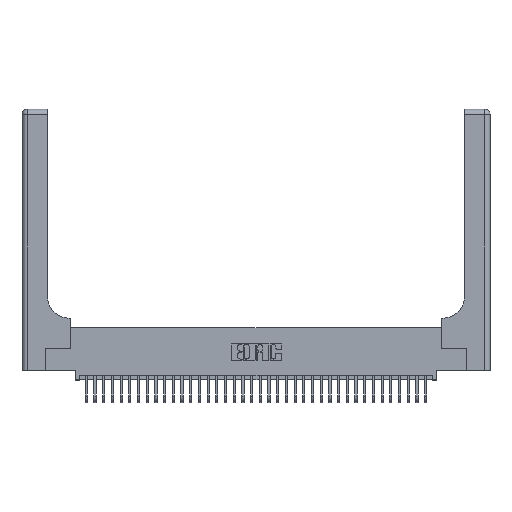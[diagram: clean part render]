
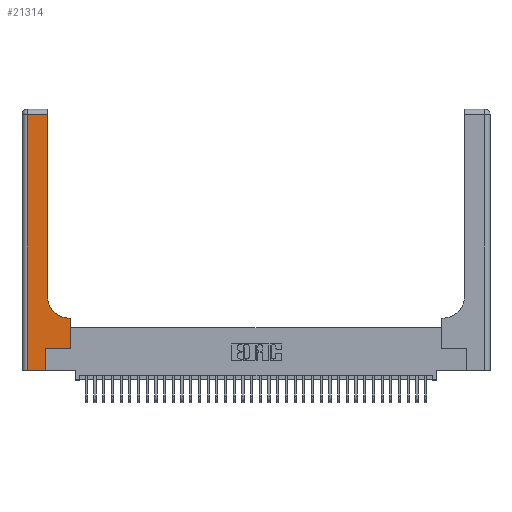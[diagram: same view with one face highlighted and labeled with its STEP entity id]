
A CAD part, top view. The second image highlights one B-rep face of the part: STEP entity #21314.
In plain terms, the highlighted planar face has unit normal (0, 0, 1).
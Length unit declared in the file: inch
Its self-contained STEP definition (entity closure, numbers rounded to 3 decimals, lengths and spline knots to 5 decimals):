
#28 = FACE_OUTER_BOUND ( 'NONE', #20406, .T. ) ;
#449 = CARTESIAN_POINT ( 'NONE',  ( 0., 3., 0.37 ) ) ;
#953 = ORIENTED_EDGE ( 'NONE', *, *, #19764, .T. ) ;
#1209 = CARTESIAN_POINT ( 'NONE',  ( 0., 0., 0.37 ) ) ;
#1913 = DIRECTION ( 'NONE',  ( 1., 0., 0. ) ) ;
#3191 = ORIENTED_EDGE ( 'NONE', *, *, #21741, .T. ) ;
#3559 = LINE ( 'NONE', #14087, #33366 ) ;
#4087 = CARTESIAN_POINT ( 'NONE',  ( 0., 2.94, 0.37 ) ) ;
#4376 = ORIENTED_EDGE ( 'NONE', *, *, #20528, .T. ) ;
#5124 = CARTESIAN_POINT ( 'NONE',  ( 0.2915, 0.6, 0.37 ) ) ;
#5545 = VERTEX_POINT ( 'NONE', #21077 ) ;
#5930 = CARTESIAN_POINT ( 'NONE',  ( 0.2915, 2.94, 0.37 ) ) ;
#6393 = LINE ( 'NONE', #11416, #27361 ) ;
#6586 = DIRECTION ( 'NONE',  ( 0., 0., -1. ) ) ;
#6614 = EDGE_CURVE ( 'NONE', #27471, #26297, #6393, .T. ) ;
#7687 = CARTESIAN_POINT ( 'NONE',  ( 0.06, 2.94, 0.37 ) ) ;
#7763 = LINE ( 'NONE', #34626, #38439 ) ;
#8096 = LINE ( 'NONE', #4087, #31797 ) ;
#8111 = CARTESIAN_POINT ( 'NONE',  ( 0.269, 0.25, 0.37 ) ) ;
#8680 = DIRECTION ( 'NONE',  ( 0., -1., 0. ) ) ;
#9043 = LINE ( 'NONE', #1209, #16006 ) ;
#11416 = CARTESIAN_POINT ( 'NONE',  ( 0.2915, 3., 0.37 ) ) ;
#11934 = DIRECTION ( 'NONE',  ( 0., 0., -1. ) ) ;
#12227 = AXIS2_PLACEMENT_3D ( 'NONE', #449, #6586, #27434 ) ;
#12510 = PLANE ( 'NONE',  #12227 ) ;
#14087 = CARTESIAN_POINT ( 'NONE',  ( 0.269, 0., 0.37 ) ) ;
#14512 = CARTESIAN_POINT ( 'NONE',  ( 0.5585, 0.6, 0.37 ) ) ;
#14562 = CARTESIAN_POINT ( 'NONE',  ( 0.06, 3., 0.37 ) ) ;
#16006 = VECTOR ( 'NONE', #25162, 39.37008 ) ;
#16873 = VERTEX_POINT ( 'NONE', #14512 ) ;
#17071 = CARTESIAN_POINT ( 'NONE',  ( 0.5585, 0.25, 0.37 ) ) ;
#17239 = LINE ( 'NONE', #5124, #24204 ) ;
#18698 = CARTESIAN_POINT ( 'NONE',  ( 0.5415, 0.6, 0.37 ) ) ;
#18852 = ORIENTED_EDGE ( 'NONE', *, *, #18896, .T. ) ;
#18896 = EDGE_CURVE ( 'NONE', #38262, #16873, #36637, .T. ) ;
#19177 = EDGE_CURVE ( 'NONE', #5545, #31230, #3559, .T. ) ;
#19764 = EDGE_CURVE ( 'NONE', #31230, #38262, #7763, .T. ) ;
#20406 = EDGE_LOOP ( 'NONE', ( #28783, #24672, #3191, #26602, #38239, #953, #18852, #27258, #4376 ) ) ;
#20459 = CARTESIAN_POINT ( 'NONE',  ( 0.2915, 0.85, 0.37 ) ) ;
#20528 = EDGE_CURVE ( 'NONE', #32099, #27471, #36976, .T. ) ;
#21077 = CARTESIAN_POINT ( 'NONE',  ( 0.269, 0., 0.37 ) ) ;
#21314 = ADVANCED_FACE ( 'NONE', ( #28 ), #12510, .F. ) ;
#21741 = EDGE_CURVE ( 'NONE', #35045, #30534, #33581, .T. ) ;
#21974 = DIRECTION ( 'NONE',  ( -1., 0., 0. ) ) ;
#24204 = VECTOR ( 'NONE', #25982, 39.37008 ) ;
#24672 = ORIENTED_EDGE ( 'NONE', *, *, #27773, .T. ) ;
#25162 = DIRECTION ( 'NONE',  ( 1., 0., 0. ) ) ;
#25982 = DIRECTION ( 'NONE',  ( -1., 0., 0. ) ) ;
#26044 = DIRECTION ( 'NONE',  ( 0., 1., 0. ) ) ;
#26297 = VERTEX_POINT ( 'NONE', #5930 ) ;
#26602 = ORIENTED_EDGE ( 'NONE', *, *, #32752, .T. ) ;
#27258 = ORIENTED_EDGE ( 'NONE', *, *, #36423, .T. ) ;
#27361 = VECTOR ( 'NONE', #35105, 39.37008 ) ;
#27434 = DIRECTION ( 'NONE',  ( -1., 0., 0. ) ) ;
#27471 = VERTEX_POINT ( 'NONE', #20459 ) ;
#27773 = EDGE_CURVE ( 'NONE', #26297, #35045, #8096, .T. ) ;
#27848 = DIRECTION ( 'NONE',  ( 0., 1., 0. ) ) ;
#28693 = CARTESIAN_POINT ( 'NONE',  ( 0.06, 0., 0.37 ) ) ;
#28783 = ORIENTED_EDGE ( 'NONE', *, *, #6614, .T. ) ;
#29707 = CARTESIAN_POINT ( 'NONE',  ( 0.5415, 0.85, 0.37 ) ) ;
#30534 = VERTEX_POINT ( 'NONE', #28693 ) ;
#30823 = CARTESIAN_POINT ( 'NONE',  ( 0.5585, 0.25, 0.37 ) ) ;
#31230 = VERTEX_POINT ( 'NONE', #8111 ) ;
#31797 = VECTOR ( 'NONE', #21974, 39.37008 ) ;
#32099 = VERTEX_POINT ( 'NONE', #18698 ) ;
#32637 = DIRECTION ( 'NONE',  ( 1., 0., 0. ) ) ;
#32667 = VECTOR ( 'NONE', #8680, 39.37008 ) ;
#32752 = EDGE_CURVE ( 'NONE', #30534, #5545, #9043, .T. ) ;
#33366 = VECTOR ( 'NONE', #26044, 39.37008 ) ;
#33581 = LINE ( 'NONE', #14562, #32667 ) ;
#34283 = AXIS2_PLACEMENT_3D ( 'NONE', #29707, #11934, #32637 ) ;
#34626 = CARTESIAN_POINT ( 'NONE',  ( 0.269, 0.25, 0.37 ) ) ;
#35045 = VERTEX_POINT ( 'NONE', #7687 ) ;
#35105 = DIRECTION ( 'NONE',  ( 0., 1., 0. ) ) ;
#35717 = VECTOR ( 'NONE', #27848, 39.37008 ) ;
#36423 = EDGE_CURVE ( 'NONE', #16873, #32099, #17239, .T. ) ;
#36637 = LINE ( 'NONE', #30823, #35717 ) ;
#36976 = CIRCLE ( 'NONE', #34283, 0.25 ) ;
#38239 = ORIENTED_EDGE ( 'NONE', *, *, #19177, .T. ) ;
#38262 = VERTEX_POINT ( 'NONE', #17071 ) ;
#38439 = VECTOR ( 'NONE', #1913, 39.37008 ) ;
